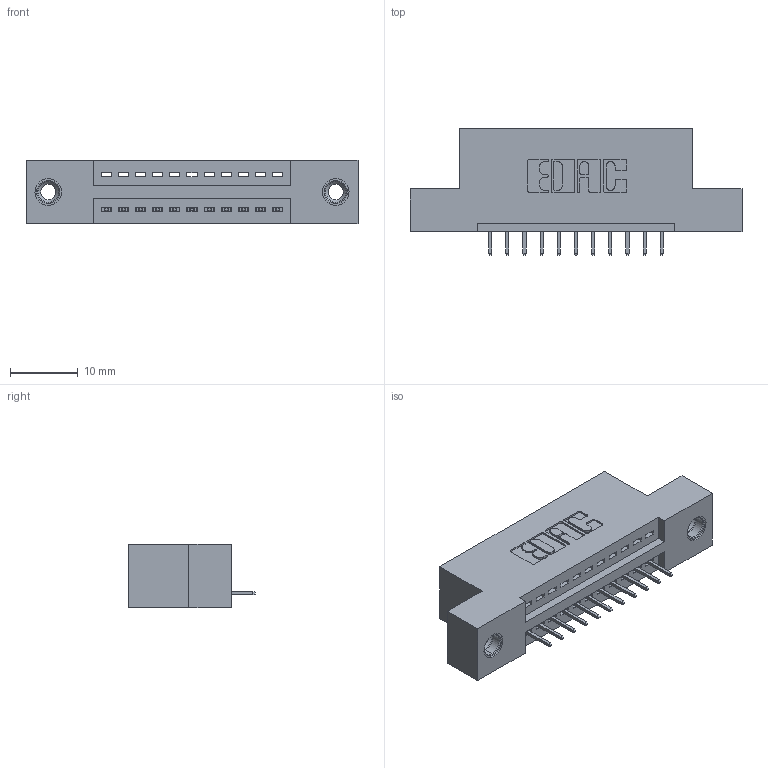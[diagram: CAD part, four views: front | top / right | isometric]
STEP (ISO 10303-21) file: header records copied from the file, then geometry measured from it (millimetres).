
FILE_DESCRIPTION (( 'STEP AP203' ), '1' );
FILE_NAME ('845-011-525-108.STEP', '2020-09-22T15:54:33', ( '' ), ( '' ), 'SwSTEP 2.0', 'SolidWorks 2020', '' );
FILE_SCHEMA (( 'CONFIG_CONTROL_DESIGN' ));
Length unit declared in the file: inch
Products named in the file (4): 845-011-525-108; 845 Part_Flush Mounting Lugs - 0.156 Dia-TI; 345-250-001_345-250-003-102; 345-292-001_345-293-125
Assembly tree (14 placements, depth 2):
  845-011-525-108
    845 Part_Flush Mounting Lugs - 0.156 Dia-TI
    345-292-001_345-293-125  x11
    345-250-001_345-250-003-102  x2
Bounding box: 49.15 x 18.72 x 9.4 mm (x, y, z)
Volume: 4362.9 mm3; surface area: 5245.9 mm2
Topology: 14 solids, 14 shells, 868 faces, 2457 edges, 1586 vertices
Faces by surface type: plane 618, cylinder 234, cone 12, torus 4
Entity records: 13712 total; most frequent: CARTESIAN_POINT 2356, ORIENTED_EDGE 2294, DIRECTION 2131, EDGE_CURVE 1147, VECTOR 955, LINE 955, VERTEX_POINT 756, AXIS2_PLACEMENT_3D 588
